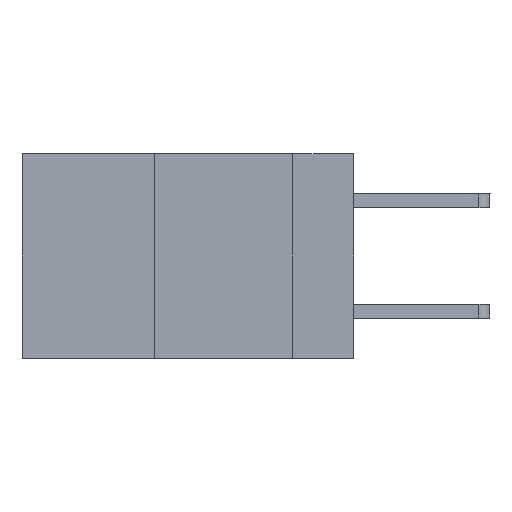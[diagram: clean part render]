
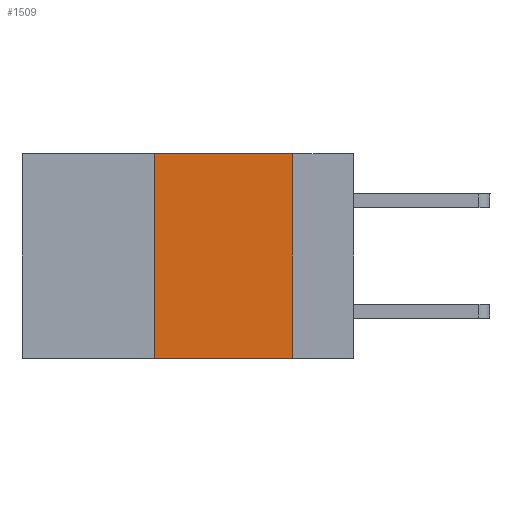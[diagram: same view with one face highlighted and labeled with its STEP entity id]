
A CAD part, left-side view. The second image highlights one B-rep face of the part: STEP entity #1509.
In plain terms, the highlighted planar face has unit normal (-1, 0, 0).
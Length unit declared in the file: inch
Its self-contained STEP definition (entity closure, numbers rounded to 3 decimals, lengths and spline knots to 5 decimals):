
#590 = DIRECTION ( 'NONE',  ( 0., -1., 0. ) ) ;
#627 = CARTESIAN_POINT ( 'NONE',  ( 0., 0.6, 0. ) ) ;
#1449 = CARTESIAN_POINT ( 'NONE',  ( 0., 0.36, 0. ) ) ;
#1509 = ADVANCED_FACE ( 'NONE', ( #10016 ), #1896, .F. ) ;
#1815 = DIRECTION ( 'NONE',  ( 0., 0., -1. ) ) ;
#1818 = DIRECTION ( 'NONE',  ( 1., 0., 0. ) ) ;
#1896 = PLANE ( 'NONE',  #7321 ) ;
#1946 = VECTOR ( 'NONE', #6272, 39.37008 ) ;
#2033 = LINE ( 'NONE', #9255, #8380 ) ;
#2686 = EDGE_CURVE ( 'NONE', #5006, #7049, #6587, .T. ) ;
#2713 = CARTESIAN_POINT ( 'NONE',  ( 0., 0.6, 0. ) ) ;
#2755 = CARTESIAN_POINT ( 'NONE',  ( 0., 0.6, -0.37 ) ) ;
#3489 = CARTESIAN_POINT ( 'NONE',  ( 0., 0.11, -0.37 ) ) ;
#3634 = ORIENTED_EDGE ( 'NONE', *, *, #10123, .F. ) ;
#4245 = ORIENTED_EDGE ( 'NONE', *, *, #2686, .F. ) ;
#4768 = VERTEX_POINT ( 'NONE', #5835 ) ;
#5006 = VERTEX_POINT ( 'NONE', #6918 ) ;
#5674 = DIRECTION ( 'NONE',  ( 0., -1., 0. ) ) ;
#5835 = CARTESIAN_POINT ( 'NONE',  ( 0., 0.36, -0.37 ) ) ;
#6135 = LINE ( 'NONE', #2755, #9420 ) ;
#6272 = DIRECTION ( 'NONE',  ( 0., 0., 1. ) ) ;
#6587 = LINE ( 'NONE', #627, #8729 ) ;
#6918 = CARTESIAN_POINT ( 'NONE',  ( 0., 0.36, 0. ) ) ;
#7049 = VERTEX_POINT ( 'NONE', #11120 ) ;
#7321 = AXIS2_PLACEMENT_3D ( 'NONE', #2713, #1818, #1815 ) ;
#7423 = ORIENTED_EDGE ( 'NONE', *, *, #11214, .T. ) ;
#7628 = EDGE_CURVE ( 'NONE', #4768, #5006, #10941, .T. ) ;
#7672 = VERTEX_POINT ( 'NONE', #3489 ) ;
#8294 = EDGE_LOOP ( 'NONE', ( #3634, #4245, #11150, #7423 ) ) ;
#8380 = VECTOR ( 'NONE', #10087, 39.37008 ) ;
#8729 = VECTOR ( 'NONE', #590, 39.37008 ) ;
#9255 = CARTESIAN_POINT ( 'NONE',  ( 0., 0.11, 0. ) ) ;
#9420 = VECTOR ( 'NONE', #5674, 39.37008 ) ;
#10016 = FACE_OUTER_BOUND ( 'NONE', #8294, .T. ) ;
#10087 = DIRECTION ( 'NONE',  ( 0., 0., -1. ) ) ;
#10123 = EDGE_CURVE ( 'NONE', #7049, #7672, #2033, .T. ) ;
#10941 = LINE ( 'NONE', #1449, #1946 ) ;
#11120 = CARTESIAN_POINT ( 'NONE',  ( 0., 0.11, 0. ) ) ;
#11150 = ORIENTED_EDGE ( 'NONE', *, *, #7628, .F. ) ;
#11214 = EDGE_CURVE ( 'NONE', #4768, #7672, #6135, .T. ) ;
